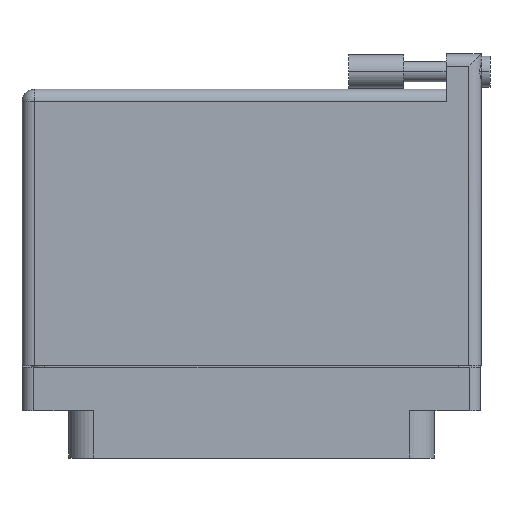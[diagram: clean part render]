
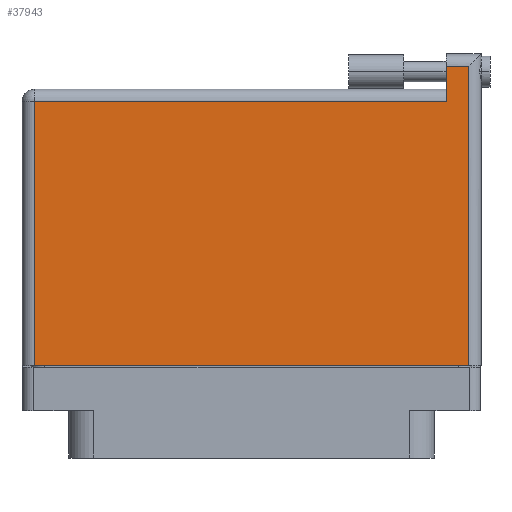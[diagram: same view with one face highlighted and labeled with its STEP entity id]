
A CAD part, front view. The second image highlights one B-rep face of the part: STEP entity #37943.
In plain terms, the highlighted face is planar.
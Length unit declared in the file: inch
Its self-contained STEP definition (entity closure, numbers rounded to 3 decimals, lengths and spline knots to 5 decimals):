
#1484 = VERTEX_POINT ( 'NONE', #9529 ) ;
#1807 = PLANE ( 'NONE',  #45107 ) ;
#2509 = FACE_OUTER_BOUND ( 'NONE', #12702, .T. ) ;
#4249 = ORIENTED_EDGE ( 'NONE', *, *, #40130, .T. ) ;
#4423 = VECTOR ( 'NONE', #12205, 39.37008 ) ;
#5130 = EDGE_CURVE ( 'NONE', #25768, #1484, #41301, .T. ) ;
#5275 = CARTESIAN_POINT ( 'NONE',  ( -1.23, -0.1, 0.4495 ) ) ;
#5619 = CARTESIAN_POINT ( 'NONE',  ( 1.103, 1.596, 0.4495 ) ) ;
#5687 = EDGE_CURVE ( 'NONE', #45093, #42578, #23428, .T. ) ;
#6863 = VECTOR ( 'NONE', #13215, 39.37008 ) ;
#9529 = CARTESIAN_POINT ( 'NONE',  ( 1.23, 1.596, 0.4495 ) ) ;
#9609 = ORIENTED_EDGE ( 'NONE', *, *, #14115, .T. ) ;
#10544 = CARTESIAN_POINT ( 'NONE',  ( 1.23, -0.1, 0.4495 ) ) ;
#11123 = VERTEX_POINT ( 'NONE', #5619 ) ;
#11855 = ORIENTED_EDGE ( 'NONE', *, *, #23388, .T. ) ;
#12205 = DIRECTION ( 'NONE',  ( -1., 0., 0. ) ) ;
#12702 = EDGE_LOOP ( 'NONE', ( #4249, #26596, #11855, #40736, #22271, #9609 ) ) ;
#13215 = DIRECTION ( 'NONE',  ( 0., -1., 0. ) ) ;
#14115 = EDGE_CURVE ( 'NONE', #42578, #24339, #17448, .T. ) ;
#16312 = CARTESIAN_POINT ( 'NONE',  ( -1.3, 1.596, 0.4495 ) ) ;
#16530 = DIRECTION ( 'NONE',  ( -1., 0., 0. ) ) ;
#16666 = CARTESIAN_POINT ( 'NONE',  ( -1.3, 1.396, 0.4495 ) ) ;
#17448 = LINE ( 'NONE', #21296, #32548 ) ;
#17690 = DIRECTION ( 'NONE',  ( 0., -1., 0. ) ) ;
#19031 = EDGE_CURVE ( 'NONE', #11123, #45093, #46251, .T. ) ;
#20517 = DIRECTION ( 'NONE',  ( -1., 0., 0. ) ) ;
#21296 = CARTESIAN_POINT ( 'NONE',  ( -1.23, -0.1, 0.4495 ) ) ;
#22271 = ORIENTED_EDGE ( 'NONE', *, *, #5687, .T. ) ;
#23388 = EDGE_CURVE ( 'NONE', #1484, #11123, #34629, .T. ) ;
#23428 = LINE ( 'NONE', #16666, #40583 ) ;
#24339 = VERTEX_POINT ( 'NONE', #5275 ) ;
#25768 = VERTEX_POINT ( 'NONE', #10544 ) ;
#26596 = ORIENTED_EDGE ( 'NONE', *, *, #5130, .T. ) ;
#27982 = VECTOR ( 'NONE', #30700, 39.37008 ) ;
#29767 = CARTESIAN_POINT ( 'NONE',  ( -1.3, -0.1, 0.4495 ) ) ;
#30700 = DIRECTION ( 'NONE',  ( 0., 1., 0. ) ) ;
#31995 = CARTESIAN_POINT ( 'NONE',  ( -1.23, 1.396, 0.4495 ) ) ;
#32548 = VECTOR ( 'NONE', #17690, 39.37008 ) ;
#33160 = DIRECTION ( 'NONE',  ( 1., 0., 0. ) ) ;
#34066 = CARTESIAN_POINT ( 'NONE',  ( 1.23, 1.666, 0.4495 ) ) ;
#34618 = DIRECTION ( 'NONE',  ( 0., 0., -1. ) ) ;
#34629 = LINE ( 'NONE', #16312, #4423 ) ;
#35170 = VECTOR ( 'NONE', #33160, 39.37008 ) ;
#35586 = LINE ( 'NONE', #29767, #35170 ) ;
#37943 = ADVANCED_FACE ( 'NONE', ( #2509 ), #1807, .F. ) ;
#38921 = CARTESIAN_POINT ( 'NONE',  ( -1.3, 1.466, 0.4495 ) ) ;
#40130 = EDGE_CURVE ( 'NONE', #24339, #25768, #35586, .T. ) ;
#40583 = VECTOR ( 'NONE', #20517, 39.37008 ) ;
#40736 = ORIENTED_EDGE ( 'NONE', *, *, #19031, .T. ) ;
#41301 = LINE ( 'NONE', #34066, #27982 ) ;
#42578 = VERTEX_POINT ( 'NONE', #31995 ) ;
#42621 = CARTESIAN_POINT ( 'NONE',  ( 1.103, 1.666, 0.4495 ) ) ;
#45093 = VERTEX_POINT ( 'NONE', #46221 ) ;
#45107 = AXIS2_PLACEMENT_3D ( 'NONE', #38921, #34618, #16530 ) ;
#46221 = CARTESIAN_POINT ( 'NONE',  ( 1.103, 1.396, 0.4495 ) ) ;
#46251 = LINE ( 'NONE', #42621, #6863 ) ;
